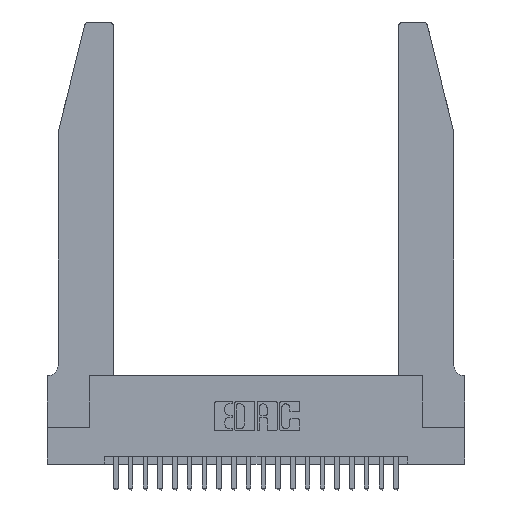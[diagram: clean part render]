
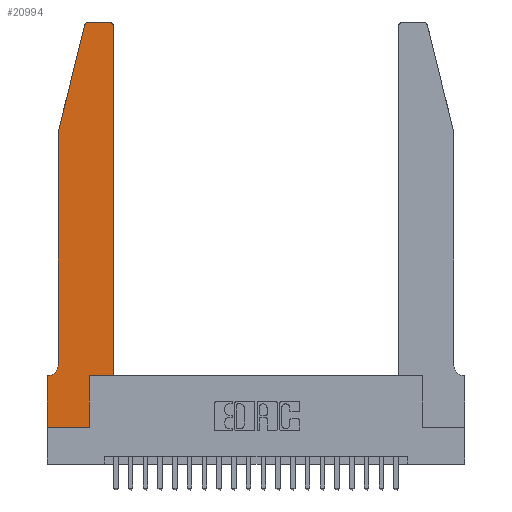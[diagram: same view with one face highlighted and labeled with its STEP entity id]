
A CAD part, top view. The second image highlights one B-rep face of the part: STEP entity #20994.
In plain terms, the highlighted planar face has unit normal (0, 0, 1).
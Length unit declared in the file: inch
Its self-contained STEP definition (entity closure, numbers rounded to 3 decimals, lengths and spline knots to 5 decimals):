
#210 = LINE ( 'NONE', #5113, #19272 ) ;
#697 = CIRCLE ( 'NONE', #21051, 0.03 ) ;
#1217 = VECTOR ( 'NONE', #1653, 39.37008 ) ;
#1228 = VECTOR ( 'NONE', #10343, 39.37008 ) ;
#1241 = CARTESIAN_POINT ( 'NONE',  ( 0.0755, 2., 0.37 ) ) ;
#1326 = DIRECTION ( 'NONE',  ( 1., 0., 0. ) ) ;
#1463 = LINE ( 'NONE', #1241, #10872 ) ;
#1653 = DIRECTION ( 'NONE',  ( -1., 0., 0. ) ) ;
#1949 = DIRECTION ( 'NONE',  ( 0., 0., -1. ) ) ;
#1980 = VERTEX_POINT ( 'NONE', #17985 ) ;
#2097 = AXIS2_PLACEMENT_3D ( 'NONE', #20563, #9847, #22271 ) ;
#2162 = CARTESIAN_POINT ( 'NONE',  ( 0., 0., 0.37 ) ) ;
#3337 = DIRECTION ( 'NONE',  ( 1., 0., 0. ) ) ;
#3709 = VERTEX_POINT ( 'NONE', #12570 ) ;
#3895 = DIRECTION ( 'NONE',  ( 0., 1., 0. ) ) ;
#4411 = VERTEX_POINT ( 'NONE', #4823 ) ;
#4823 = CARTESIAN_POINT ( 'NONE',  ( 0.0755, 2., 0.37 ) ) ;
#5113 = CARTESIAN_POINT ( 'NONE',  ( 0.2865, 0.35, 0.37 ) ) ;
#5520 = AXIS2_PLACEMENT_3D ( 'NONE', #13013, #1949, #14857 ) ;
#5634 = CARTESIAN_POINT ( 'NONE',  ( 0.284, 2.75, 0.37 ) ) ;
#5646 = LINE ( 'NONE', #12119, #1228 ) ;
#6622 = CARTESIAN_POINT ( 'NONE',  ( 0.2865, 0., 0.37 ) ) ;
#6914 = CARTESIAN_POINT ( 'NONE',  ( 0.4205, 2.72, 0.37 ) ) ;
#7030 = DIRECTION ( 'NONE',  ( 0., 1., 0. ) ) ;
#7214 = EDGE_CURVE ( 'NONE', #12996, #8157, #20681, .T. ) ;
#7273 = CARTESIAN_POINT ( 'NONE',  ( 0.4205, 2.75, 0.37 ) ) ;
#7562 = CARTESIAN_POINT ( 'NONE',  ( 0.4505, 0.35, 0.37 ) ) ;
#8030 = EDGE_CURVE ( 'NONE', #12942, #4411, #5646, .T. ) ;
#8157 = VERTEX_POINT ( 'NONE', #12426 ) ;
#8472 = VERTEX_POINT ( 'NONE', #15179 ) ;
#8613 = CARTESIAN_POINT ( 'NONE',  ( 0., 0., 0.37 ) ) ;
#8812 = DIRECTION ( 'NONE',  ( 1., 0., 0. ) ) ;
#9038 = LINE ( 'NONE', #8613, #13184 ) ;
#9439 = LINE ( 'NONE', #21052, #13604 ) ;
#9847 = DIRECTION ( 'NONE',  ( 0., 0., 1. ) ) ;
#9948 = CARTESIAN_POINT ( 'NONE',  ( 0.0055, 0.35, 0.37 ) ) ;
#9999 = CARTESIAN_POINT ( 'NONE',  ( 0.4505, 2.72, 0.37 ) ) ;
#10343 = DIRECTION ( 'NONE',  ( -0.239, -0.971, 0. ) ) ;
#10369 = DIRECTION ( 'NONE',  ( 0., -1., 0. ) ) ;
#10405 = ORIENTED_EDGE ( 'NONE', *, *, #10749, .T. ) ;
#10411 = VERTEX_POINT ( 'NONE', #6622 ) ;
#10619 = DIRECTION ( 'NONE',  ( 0., -1., 0. ) ) ;
#10700 = CARTESIAN_POINT ( 'NONE',  ( 0., 0.35, 0.37 ) ) ;
#10749 = EDGE_CURVE ( 'NONE', #8472, #3709, #9439, .T. ) ;
#10858 = EDGE_CURVE ( 'NONE', #4411, #1980, #1463, .T. ) ;
#10872 = VECTOR ( 'NONE', #10619, 39.37008 ) ;
#11041 = VERTEX_POINT ( 'NONE', #2162 ) ;
#11211 = LINE ( 'NONE', #12757, #20162 ) ;
#11333 = LINE ( 'NONE', #15678, #15534 ) ;
#11373 = EDGE_CURVE ( 'NONE', #10411, #8472, #210, .T. ) ;
#11628 = ORIENTED_EDGE ( 'NONE', *, *, #13293, .T. ) ;
#11786 = VERTEX_POINT ( 'NONE', #9999 ) ;
#11848 = LINE ( 'NONE', #7562, #15518 ) ;
#12119 = CARTESIAN_POINT ( 'NONE',  ( 0.0755, 2., 0.37 ) ) ;
#12290 = ORIENTED_EDGE ( 'NONE', *, *, #18648, .T. ) ;
#12426 = CARTESIAN_POINT ( 'NONE',  ( 0., 0.35, 0.37 ) ) ;
#12451 = DIRECTION ( 'NONE',  ( 0., 0., 1. ) ) ;
#12570 = CARTESIAN_POINT ( 'NONE',  ( 0.4505, 0.35, 0.37 ) ) ;
#12616 = ORIENTED_EDGE ( 'NONE', *, *, #17126, .T. ) ;
#12757 = CARTESIAN_POINT ( 'NONE',  ( 0., 0., 0.37 ) ) ;
#12828 = FACE_OUTER_BOUND ( 'NONE', #18508, .T. ) ;
#12886 = ORIENTED_EDGE ( 'NONE', *, *, #7214, .T. ) ;
#12942 = VERTEX_POINT ( 'NONE', #18767 ) ;
#12996 = VERTEX_POINT ( 'NONE', #9948 ) ;
#13013 = CARTESIAN_POINT ( 'NONE',  ( 0.0055, 0.42, 0.37 ) ) ;
#13184 = VECTOR ( 'NONE', #10369, 39.37008 ) ;
#13293 = EDGE_CURVE ( 'NONE', #19787, #22641, #11333, .T. ) ;
#13590 = EDGE_CURVE ( 'NONE', #1980, #12996, #19479, .T. ) ;
#13604 = VECTOR ( 'NONE', #22766, 39.37008 ) ;
#14370 = EDGE_CURVE ( 'NONE', #8157, #11041, #9038, .T. ) ;
#14790 = ORIENTED_EDGE ( 'NONE', *, *, #10858, .T. ) ;
#14857 = DIRECTION ( 'NONE',  ( -1., 0., 0. ) ) ;
#15179 = CARTESIAN_POINT ( 'NONE',  ( 0.2865, 0.35, 0.37 ) ) ;
#15499 = ORIENTED_EDGE ( 'NONE', *, *, #17666, .T. ) ;
#15518 = VECTOR ( 'NONE', #3895, 39.37008 ) ;
#15534 = VECTOR ( 'NONE', #22738, 39.37008 ) ;
#15678 = CARTESIAN_POINT ( 'NONE',  ( 0.2605, 2.75, 0.37 ) ) ;
#16683 = AXIS2_PLACEMENT_3D ( 'NONE', #10700, #12451, #1326 ) ;
#17126 = EDGE_CURVE ( 'NONE', #22641, #12942, #22425, .T. ) ;
#17210 = ORIENTED_EDGE ( 'NONE', *, *, #23104, .T. ) ;
#17666 = EDGE_CURVE ( 'NONE', #3709, #11786, #11848, .T. ) ;
#17834 = ORIENTED_EDGE ( 'NONE', *, *, #13590, .T. ) ;
#17985 = CARTESIAN_POINT ( 'NONE',  ( 0.0755, 0.42, 0.37 ) ) ;
#18508 = EDGE_LOOP ( 'NONE', ( #11628, #12616, #20781, #14790, #17834, #12886, #21947, #17210, #21656, #10405, #15499, #12290 ) ) ;
#18648 = EDGE_CURVE ( 'NONE', #11786, #19787, #697, .T. ) ;
#18767 = CARTESIAN_POINT ( 'NONE',  ( 0.25487, 2.72718, 0.37 ) ) ;
#19272 = VECTOR ( 'NONE', #7030, 39.37008 ) ;
#19479 = CIRCLE ( 'NONE', #5520, 0.07 ) ;
#19594 = DIRECTION ( 'NONE',  ( 0., 0., 1. ) ) ;
#19787 = VERTEX_POINT ( 'NONE', #7273 ) ;
#19927 = CARTESIAN_POINT ( 'NONE',  ( 0.0755, 0.35, 0.37 ) ) ;
#20162 = VECTOR ( 'NONE', #3337, 39.37008 ) ;
#20563 = CARTESIAN_POINT ( 'NONE',  ( 0.284, 2.72, 0.37 ) ) ;
#20681 = LINE ( 'NONE', #19927, #1217 ) ;
#20781 = ORIENTED_EDGE ( 'NONE', *, *, #8030, .T. ) ;
#20994 = ADVANCED_FACE ( 'NONE', ( #12828 ), #21354, .T. ) ;
#21051 = AXIS2_PLACEMENT_3D ( 'NONE', #6914, #19594, #8812 ) ;
#21052 = CARTESIAN_POINT ( 'NONE',  ( 0.4505, 0.35, 0.37 ) ) ;
#21354 = PLANE ( 'NONE',  #16683 ) ;
#21656 = ORIENTED_EDGE ( 'NONE', *, *, #11373, .T. ) ;
#21947 = ORIENTED_EDGE ( 'NONE', *, *, #14370, .T. ) ;
#22271 = DIRECTION ( 'NONE',  ( 1., 0., 0. ) ) ;
#22425 = CIRCLE ( 'NONE', #2097, 0.03 ) ;
#22641 = VERTEX_POINT ( 'NONE', #5634 ) ;
#22738 = DIRECTION ( 'NONE',  ( -1., 0., 0. ) ) ;
#22766 = DIRECTION ( 'NONE',  ( 1., 0., 0. ) ) ;
#23104 = EDGE_CURVE ( 'NONE', #11041, #10411, #11211, .T. ) ;
